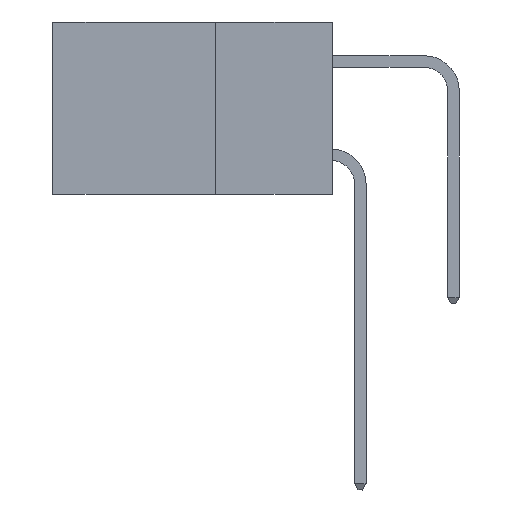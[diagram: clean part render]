
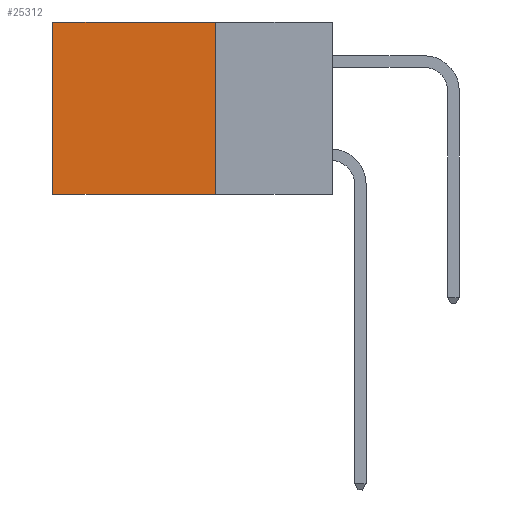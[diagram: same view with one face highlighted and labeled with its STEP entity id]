
A CAD part, left-side view. The second image highlights one B-rep face of the part: STEP entity #25312.
In plain terms, the highlighted planar face has unit normal (-1, 0, 0).
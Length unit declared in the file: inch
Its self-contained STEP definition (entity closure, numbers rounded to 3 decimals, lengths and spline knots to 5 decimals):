
#424 = ORIENTED_EDGE ( 'NONE', *, *, #15748, .F. ) ;
#1390 = EDGE_CURVE ( 'NONE', #16638, #30105, #26077, .T. ) ;
#1939 = DIRECTION ( 'NONE',  ( 1., 0., 0. ) ) ;
#6031 = CARTESIAN_POINT ( 'NONE',  ( 0.298, 0.6, -0.37 ) ) ;
#7449 = DIRECTION ( 'NONE',  ( 0., 1., 0. ) ) ;
#8034 = LINE ( 'NONE', #12348, #11371 ) ;
#9717 = VECTOR ( 'NONE', #11618, 39.37008 ) ;
#10867 = CARTESIAN_POINT ( 'NONE',  ( 0.298, 0.6, 0. ) ) ;
#11054 = EDGE_CURVE ( 'NONE', #13888, #24015, #16223, .T. ) ;
#11297 = CARTESIAN_POINT ( 'NONE',  ( 0.298, 0.25, 0. ) ) ;
#11371 = VECTOR ( 'NONE', #7449, 39.37008 ) ;
#11618 = DIRECTION ( 'NONE',  ( 0., 1., 0. ) ) ;
#12227 = FACE_OUTER_BOUND ( 'NONE', #28788, .T. ) ;
#12348 = CARTESIAN_POINT ( 'NONE',  ( 0.298, 0.25, 0. ) ) ;
#13642 = PLANE ( 'NONE',  #22561 ) ;
#13888 = VERTEX_POINT ( 'NONE', #11297 ) ;
#15748 = EDGE_CURVE ( 'NONE', #24015, #30105, #16050, .T. ) ;
#16050 = LINE ( 'NONE', #16224, #9717 ) ;
#16223 = LINE ( 'NONE', #24225, #29728 ) ;
#16224 = CARTESIAN_POINT ( 'NONE',  ( 0.298, 0.25, -0.37 ) ) ;
#16638 = VERTEX_POINT ( 'NONE', #27417 ) ;
#17740 = CARTESIAN_POINT ( 'NONE',  ( 0.298, 0.25, -0.37 ) ) ;
#20298 = DIRECTION ( 'NONE',  ( 0., 0., -1. ) ) ;
#20992 = EDGE_CURVE ( 'NONE', #13888, #16638, #8034, .T. ) ;
#22561 = AXIS2_PLACEMENT_3D ( 'NONE', #25592, #1939, #25892 ) ;
#22973 = ORIENTED_EDGE ( 'NONE', *, *, #11054, .F. ) ;
#24015 = VERTEX_POINT ( 'NONE', #17740 ) ;
#24225 = CARTESIAN_POINT ( 'NONE',  ( 0.298, 0.25, 0. ) ) ;
#25312 = ADVANCED_FACE ( 'NONE', ( #12227 ), #13642, .F. ) ;
#25592 = CARTESIAN_POINT ( 'NONE',  ( 0.298, 0.25, 0. ) ) ;
#25892 = DIRECTION ( 'NONE',  ( 0., 0., -1. ) ) ;
#26077 = LINE ( 'NONE', #10867, #27221 ) ;
#27071 = DIRECTION ( 'NONE',  ( 0., 0., -1. ) ) ;
#27221 = VECTOR ( 'NONE', #20298, 39.37008 ) ;
#27417 = CARTESIAN_POINT ( 'NONE',  ( 0.298, 0.6, 0. ) ) ;
#27956 = ORIENTED_EDGE ( 'NONE', *, *, #1390, .T. ) ;
#28788 = EDGE_LOOP ( 'NONE', ( #27956, #424, #22973, #30353 ) ) ;
#29728 = VECTOR ( 'NONE', #27071, 39.37008 ) ;
#30105 = VERTEX_POINT ( 'NONE', #6031 ) ;
#30353 = ORIENTED_EDGE ( 'NONE', *, *, #20992, .T. ) ;
